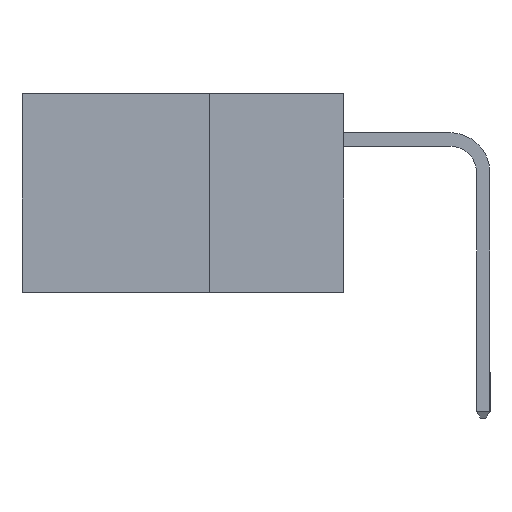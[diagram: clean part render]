
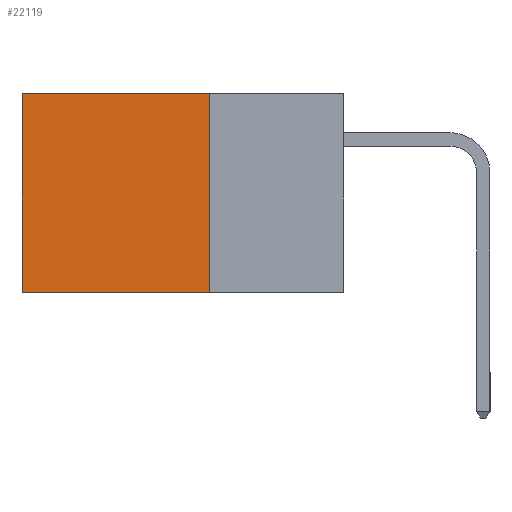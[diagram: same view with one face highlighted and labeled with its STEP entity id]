
A CAD part, left-side view. The second image highlights one B-rep face of the part: STEP entity #22119.
In plain terms, the highlighted planar face has unit normal (-1, 0, 0).
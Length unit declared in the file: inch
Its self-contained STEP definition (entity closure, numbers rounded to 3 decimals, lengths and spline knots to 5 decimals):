
#334 = VECTOR ( 'NONE', #6545, 39.37008 ) ;
#575 = DIRECTION ( 'NONE',  ( 0., 0., -1. ) ) ;
#894 = CARTESIAN_POINT ( 'NONE',  ( 0.2615, 0.6, 0. ) ) ;
#1407 = VERTEX_POINT ( 'NONE', #23701 ) ;
#1554 = VECTOR ( 'NONE', #575, 39.37008 ) ;
#1892 = EDGE_LOOP ( 'NONE', ( #23397, #7450, #16828, #22367 ) ) ;
#1963 = EDGE_CURVE ( 'NONE', #4394, #1407, #21844, .T. ) ;
#2414 = CARTESIAN_POINT ( 'NONE',  ( 0.2615, 0.25, -0.37 ) ) ;
#4394 = VERTEX_POINT ( 'NONE', #894 ) ;
#4466 = AXIS2_PLACEMENT_3D ( 'NONE', #16504, #22538, #14649 ) ;
#5054 = EDGE_CURVE ( 'NONE', #15207, #18511, #6100, .T. ) ;
#5685 = EDGE_CURVE ( 'NONE', #15207, #4394, #8149, .T. ) ;
#6100 = LINE ( 'NONE', #2414, #1554 ) ;
#6266 = CARTESIAN_POINT ( 'NONE',  ( 0.2615, 0.25, 0. ) ) ;
#6545 = DIRECTION ( 'NONE',  ( 0., 0., -1. ) ) ;
#7245 = VECTOR ( 'NONE', #23004, 39.37008 ) ;
#7450 = ORIENTED_EDGE ( 'NONE', *, *, #20502, .F. ) ;
#8149 = LINE ( 'NONE', #6266, #11033 ) ;
#8251 = CARTESIAN_POINT ( 'NONE',  ( 0.2615, 0.25, 0. ) ) ;
#11033 = VECTOR ( 'NONE', #13824, 39.37008 ) ;
#12122 = CARTESIAN_POINT ( 'NONE',  ( 0.2615, 0.6, -0.37 ) ) ;
#13824 = DIRECTION ( 'NONE',  ( 0., 1., 0. ) ) ;
#14649 = DIRECTION ( 'NONE',  ( 0., 0., -1. ) ) ;
#15207 = VERTEX_POINT ( 'NONE', #8251 ) ;
#15501 = CARTESIAN_POINT ( 'NONE',  ( 0.2615, 0.25, -0.37 ) ) ;
#16504 = CARTESIAN_POINT ( 'NONE',  ( 0.2615, 0.25, -0.37 ) ) ;
#16828 = ORIENTED_EDGE ( 'NONE', *, *, #5054, .F. ) ;
#18239 = PLANE ( 'NONE',  #4466 ) ;
#18511 = VERTEX_POINT ( 'NONE', #23063 ) ;
#20502 = EDGE_CURVE ( 'NONE', #18511, #1407, #21064, .T. ) ;
#21064 = LINE ( 'NONE', #15501, #7245 ) ;
#21844 = LINE ( 'NONE', #12122, #334 ) ;
#22039 = FACE_OUTER_BOUND ( 'NONE', #1892, .T. ) ;
#22119 = ADVANCED_FACE ( 'NONE', ( #22039 ), #18239, .F. ) ;
#22367 = ORIENTED_EDGE ( 'NONE', *, *, #5685, .T. ) ;
#22538 = DIRECTION ( 'NONE',  ( 1., 0., 0. ) ) ;
#23004 = DIRECTION ( 'NONE',  ( 0., 1., 0. ) ) ;
#23063 = CARTESIAN_POINT ( 'NONE',  ( 0.2615, 0.25, -0.37 ) ) ;
#23397 = ORIENTED_EDGE ( 'NONE', *, *, #1963, .T. ) ;
#23701 = CARTESIAN_POINT ( 'NONE',  ( 0.2615, 0.6, -0.37 ) ) ;
